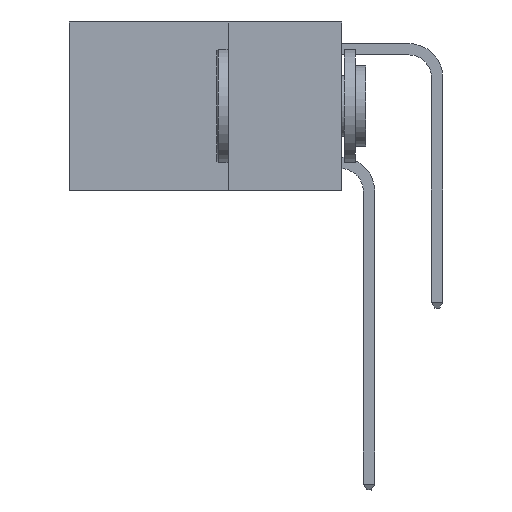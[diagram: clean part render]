
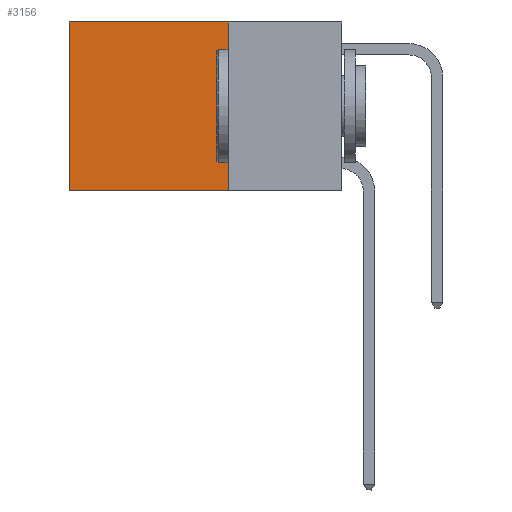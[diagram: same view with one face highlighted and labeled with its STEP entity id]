
A CAD part, left-side view. The second image highlights one B-rep face of the part: STEP entity #3156.
In plain terms, the highlighted planar face has unit normal (-1, 0, 0).
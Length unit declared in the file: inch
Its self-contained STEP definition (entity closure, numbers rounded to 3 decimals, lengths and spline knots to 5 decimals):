
#978 = ORIENTED_EDGE ( 'NONE', *, *, #6373, .T. ) ;
#2022 = DIRECTION ( 'NONE',  ( 1., 0., 0. ) ) ;
#2194 = CARTESIAN_POINT ( 'NONE',  ( 0.2625, 0.25, 0. ) ) ;
#2569 = CARTESIAN_POINT ( 'NONE',  ( 0.2625, 0.6, -0.37 ) ) ;
#3156 = ADVANCED_FACE ( 'NONE', ( #14326 ), #3604, .F. ) ;
#3236 = ORIENTED_EDGE ( 'NONE', *, *, #12871, .F. ) ;
#3544 = CARTESIAN_POINT ( 'NONE',  ( 0.2625, 0.25, 0. ) ) ;
#3604 = PLANE ( 'NONE',  #13628 ) ;
#3607 = CARTESIAN_POINT ( 'NONE',  ( 0.2625, 0.25, 0. ) ) ;
#4548 = VERTEX_POINT ( 'NONE', #14392 ) ;
#5350 = LINE ( 'NONE', #16579, #15033 ) ;
#6041 = DIRECTION ( 'NONE',  ( 0., 1., 0. ) ) ;
#6087 = VECTOR ( 'NONE', #13034, 39.37008 ) ;
#6227 = VERTEX_POINT ( 'NONE', #15169 ) ;
#6373 = EDGE_CURVE ( 'NONE', #11953, #6227, #9811, .T. ) ;
#7037 = CARTESIAN_POINT ( 'NONE',  ( 0.2625, 0.25, 0. ) ) ;
#7085 = DIRECTION ( 'NONE',  ( 0., 1., 0. ) ) ;
#7318 = VECTOR ( 'NONE', #17310, 39.37008 ) ;
#9683 = LINE ( 'NONE', #3607, #6087 ) ;
#9811 = LINE ( 'NONE', #7037, #13586 ) ;
#10110 = EDGE_CURVE ( 'NONE', #11953, #4548, #9683, .T. ) ;
#10518 = LINE ( 'NONE', #11865, #7318 ) ;
#10697 = EDGE_CURVE ( 'NONE', #6227, #14635, #10518, .T. ) ;
#11628 = ORIENTED_EDGE ( 'NONE', *, *, #10697, .T. ) ;
#11865 = CARTESIAN_POINT ( 'NONE',  ( 0.2625, 0.6, 0. ) ) ;
#11953 = VERTEX_POINT ( 'NONE', #2194 ) ;
#12871 = EDGE_CURVE ( 'NONE', #4548, #14635, #5350, .T. ) ;
#13034 = DIRECTION ( 'NONE',  ( 0., 0., -1. ) ) ;
#13586 = VECTOR ( 'NONE', #6041, 39.37008 ) ;
#13590 = EDGE_LOOP ( 'NONE', ( #11628, #3236, #16714, #978 ) ) ;
#13628 = AXIS2_PLACEMENT_3D ( 'NONE', #3544, #2022, #16864 ) ;
#14326 = FACE_OUTER_BOUND ( 'NONE', #13590, .T. ) ;
#14392 = CARTESIAN_POINT ( 'NONE',  ( 0.2625, 0.25, -0.37 ) ) ;
#14635 = VERTEX_POINT ( 'NONE', #2569 ) ;
#15033 = VECTOR ( 'NONE', #7085, 39.37008 ) ;
#15169 = CARTESIAN_POINT ( 'NONE',  ( 0.2625, 0.6, 0. ) ) ;
#16579 = CARTESIAN_POINT ( 'NONE',  ( 0.2625, 0.25, -0.37 ) ) ;
#16714 = ORIENTED_EDGE ( 'NONE', *, *, #10110, .F. ) ;
#16864 = DIRECTION ( 'NONE',  ( 0., 0., -1. ) ) ;
#17310 = DIRECTION ( 'NONE',  ( 0., 0., -1. ) ) ;
